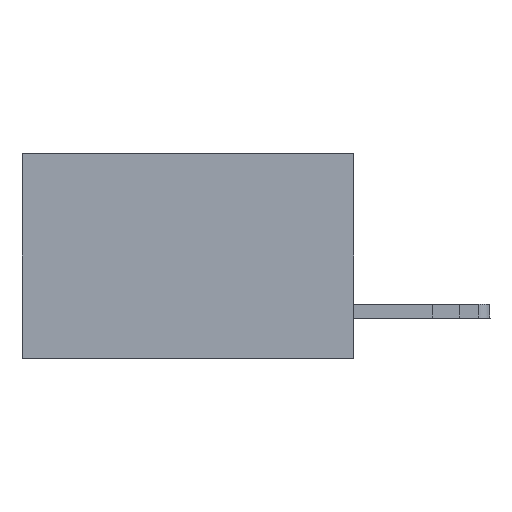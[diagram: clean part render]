
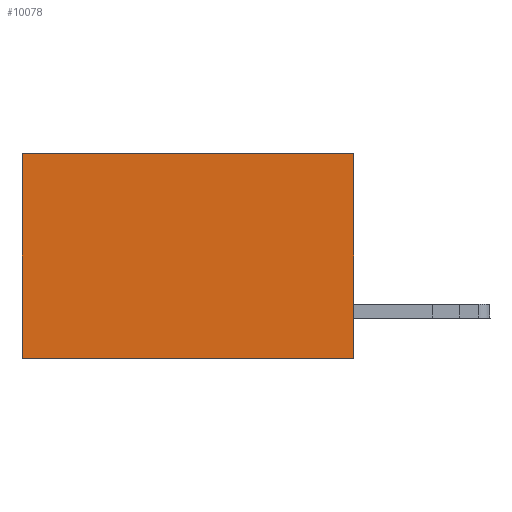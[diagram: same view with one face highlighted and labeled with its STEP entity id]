
A CAD part, left-side view. The second image highlights one B-rep face of the part: STEP entity #10078.
In plain terms, the highlighted planar face has unit normal (-1, 0, 0).
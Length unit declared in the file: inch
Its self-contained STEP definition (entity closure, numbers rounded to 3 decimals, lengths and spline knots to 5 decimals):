
#198 = ORIENTED_EDGE ( 'NONE', *, *, #891, .F. ) ;
#891 = EDGE_CURVE ( 'NONE', #22535, #22089, #25694, .T. ) ;
#1102 = LINE ( 'NONE', #19804, #11008 ) ;
#1949 = EDGE_LOOP ( 'NONE', ( #7347, #198, #22459, #9052 ) ) ;
#2042 = FACE_OUTER_BOUND ( 'NONE', #1949, .T. ) ;
#2424 = LINE ( 'NONE', #22358, #22865 ) ;
#2836 = CARTESIAN_POINT ( 'NONE',  ( 0.2875, 0., 0. ) ) ;
#3612 = VERTEX_POINT ( 'NONE', #10057 ) ;
#3716 = DIRECTION ( 'NONE',  ( 0., 0., -1. ) ) ;
#3728 = EDGE_CURVE ( 'NONE', #3612, #22535, #1102, .T. ) ;
#4049 = VECTOR ( 'NONE', #16561, 39.37008 ) ;
#4861 = DIRECTION ( 'NONE',  ( 1., 0., 0. ) ) ;
#5255 = AXIS2_PLACEMENT_3D ( 'NONE', #2836, #4861, #18663 ) ;
#6556 = DIRECTION ( 'NONE',  ( 0., 1., 0. ) ) ;
#7347 = ORIENTED_EDGE ( 'NONE', *, *, #24672, .T. ) ;
#7398 = CARTESIAN_POINT ( 'NONE',  ( 0.2875, 0.6, -0.37 ) ) ;
#7687 = CARTESIAN_POINT ( 'NONE',  ( 0.2875, 0.6, 0. ) ) ;
#8691 = DIRECTION ( 'NONE',  ( 0., 0., -1. ) ) ;
#9052 = ORIENTED_EDGE ( 'NONE', *, *, #21843, .T. ) ;
#10057 = CARTESIAN_POINT ( 'NONE',  ( 0.2875, 0., 0. ) ) ;
#10078 = ADVANCED_FACE ( 'NONE', ( #2042 ), #14669, .F. ) ;
#11008 = VECTOR ( 'NONE', #8691, 39.37008 ) ;
#11126 = CARTESIAN_POINT ( 'NONE',  ( 0.2875, 0., -0.37 ) ) ;
#14669 = PLANE ( 'NONE',  #5255 ) ;
#16561 = DIRECTION ( 'NONE',  ( 0., 1., 0. ) ) ;
#18362 = LINE ( 'NONE', #7687, #19007 ) ;
#18663 = DIRECTION ( 'NONE',  ( 0., 0., -1. ) ) ;
#18780 = CARTESIAN_POINT ( 'NONE',  ( 0.2875, 0., -0.37 ) ) ;
#18899 = CARTESIAN_POINT ( 'NONE',  ( 0.2875, 0.6, 0. ) ) ;
#19007 = VECTOR ( 'NONE', #3716, 39.37008 ) ;
#19804 = CARTESIAN_POINT ( 'NONE',  ( 0.2875, 0., 0. ) ) ;
#21843 = EDGE_CURVE ( 'NONE', #3612, #21995, #2424, .T. ) ;
#21995 = VERTEX_POINT ( 'NONE', #18899 ) ;
#22089 = VERTEX_POINT ( 'NONE', #7398 ) ;
#22358 = CARTESIAN_POINT ( 'NONE',  ( 0.2875, 0., 0. ) ) ;
#22459 = ORIENTED_EDGE ( 'NONE', *, *, #3728, .F. ) ;
#22535 = VERTEX_POINT ( 'NONE', #18780 ) ;
#22865 = VECTOR ( 'NONE', #6556, 39.37008 ) ;
#24672 = EDGE_CURVE ( 'NONE', #21995, #22089, #18362, .T. ) ;
#25694 = LINE ( 'NONE', #11126, #4049 ) ;
